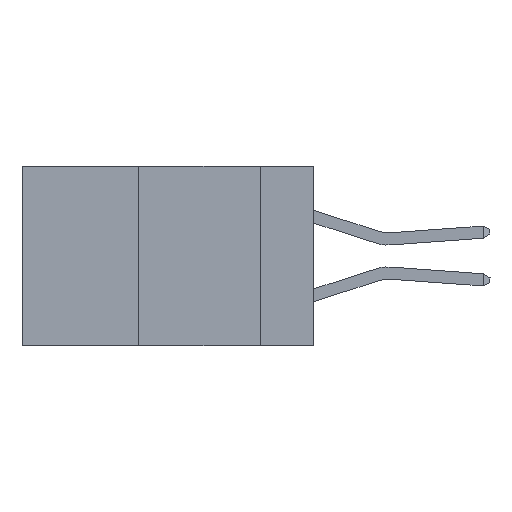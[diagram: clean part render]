
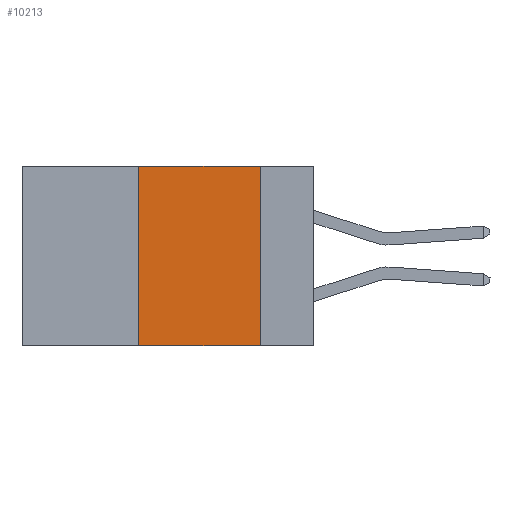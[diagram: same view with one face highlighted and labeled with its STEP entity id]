
A CAD part, left-side view. The second image highlights one B-rep face of the part: STEP entity #10213.
In plain terms, the highlighted planar face has unit normal (-1, 0, 0).
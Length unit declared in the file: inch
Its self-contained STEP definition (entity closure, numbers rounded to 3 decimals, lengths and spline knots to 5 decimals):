
#41 = VERTEX_POINT ( 'NONE', #6401 ) ;
#146 = ORIENTED_EDGE ( 'NONE', *, *, #681, .T. ) ;
#271 = CARTESIAN_POINT ( 'NONE',  ( 0., 0.36, 0. ) ) ;
#589 = ORIENTED_EDGE ( 'NONE', *, *, #10050, .F. ) ;
#681 = EDGE_CURVE ( 'NONE', #10854, #41, #11720, .T. ) ;
#1022 = DIRECTION ( 'NONE',  ( 0., 0., -1. ) ) ;
#2245 = VECTOR ( 'NONE', #11865, 39.37008 ) ;
#2640 = CARTESIAN_POINT ( 'NONE',  ( 0., 0.6, 0. ) ) ;
#2868 = CARTESIAN_POINT ( 'NONE',  ( 0., 0.36, 0. ) ) ;
#2983 = ORIENTED_EDGE ( 'NONE', *, *, #15292, .F. ) ;
#3811 = VERTEX_POINT ( 'NONE', #11374 ) ;
#4353 = CARTESIAN_POINT ( 'NONE',  ( 0., 0.36, -0.37 ) ) ;
#4453 = DIRECTION ( 'NONE',  ( 0., 0., -1. ) ) ;
#4679 = DIRECTION ( 'NONE',  ( 0., 0., 1. ) ) ;
#5410 = LINE ( 'NONE', #17958, #14241 ) ;
#5521 = AXIS2_PLACEMENT_3D ( 'NONE', #2640, #15006, #4453 ) ;
#6401 = CARTESIAN_POINT ( 'NONE',  ( 0., 0.11, -0.37 ) ) ;
#7112 = LINE ( 'NONE', #16865, #15284 ) ;
#9032 = VERTEX_POINT ( 'NONE', #271 ) ;
#9762 = PLANE ( 'NONE',  #5521 ) ;
#10050 = EDGE_CURVE ( 'NONE', #9032, #3811, #5410, .T. ) ;
#10213 = ADVANCED_FACE ( 'NONE', ( #15016 ), #9762, .F. ) ;
#10854 = VERTEX_POINT ( 'NONE', #4353 ) ;
#11075 = DIRECTION ( 'NONE',  ( 0., -1., 0. ) ) ;
#11374 = CARTESIAN_POINT ( 'NONE',  ( 0., 0.11, 0. ) ) ;
#11720 = LINE ( 'NONE', #19526, #2245 ) ;
#11865 = DIRECTION ( 'NONE',  ( 0., -1., 0. ) ) ;
#14241 = VECTOR ( 'NONE', #11075, 39.37008 ) ;
#14251 = LINE ( 'NONE', #2868, #17739 ) ;
#15006 = DIRECTION ( 'NONE',  ( 1., 0., 0. ) ) ;
#15016 = FACE_OUTER_BOUND ( 'NONE', #18865, .T. ) ;
#15284 = VECTOR ( 'NONE', #1022, 39.37008 ) ;
#15292 = EDGE_CURVE ( 'NONE', #3811, #41, #7112, .T. ) ;
#15531 = ORIENTED_EDGE ( 'NONE', *, *, #22233, .F. ) ;
#16865 = CARTESIAN_POINT ( 'NONE',  ( 0., 0.11, 0. ) ) ;
#17739 = VECTOR ( 'NONE', #4679, 39.37008 ) ;
#17958 = CARTESIAN_POINT ( 'NONE',  ( 0., 0.6, 0. ) ) ;
#18865 = EDGE_LOOP ( 'NONE', ( #2983, #589, #15531, #146 ) ) ;
#19526 = CARTESIAN_POINT ( 'NONE',  ( 0., 0.6, -0.37 ) ) ;
#22233 = EDGE_CURVE ( 'NONE', #10854, #9032, #14251, .T. ) ;
